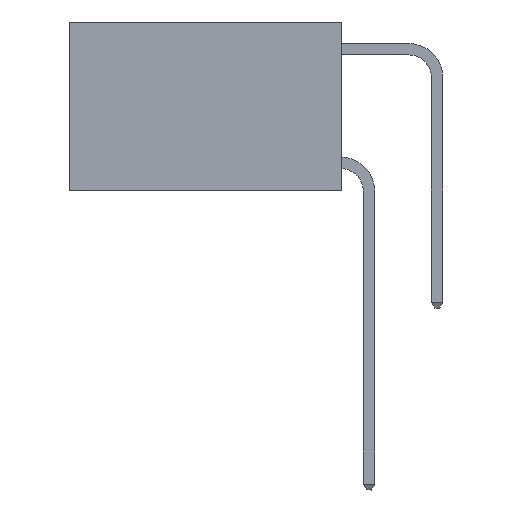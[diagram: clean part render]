
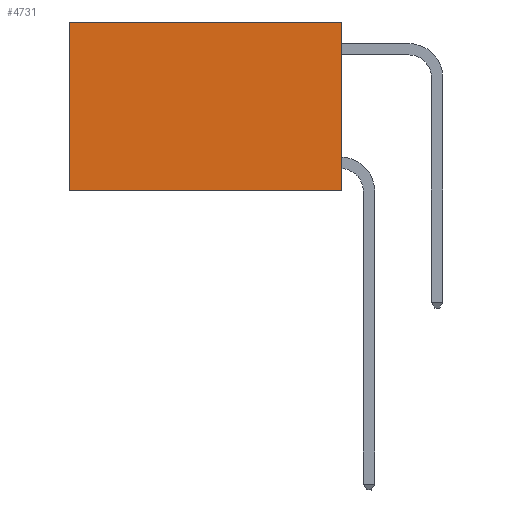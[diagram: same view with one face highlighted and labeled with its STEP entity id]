
A CAD part, left-side view. The second image highlights one B-rep face of the part: STEP entity #4731.
In plain terms, the highlighted planar face has unit normal (-1, 0, 0).
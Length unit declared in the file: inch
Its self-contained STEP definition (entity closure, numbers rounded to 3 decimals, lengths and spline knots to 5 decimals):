
#250 = VECTOR ( 'NONE', #14579, 39.37008 ) ;
#752 = CARTESIAN_POINT ( 'NONE',  ( 0.2625, 0., 0. ) ) ;
#1429 = CARTESIAN_POINT ( 'NONE',  ( 0.2625, 0.6, 0. ) ) ;
#2298 = EDGE_CURVE ( 'NONE', #16656, #6721, #19613, .T. ) ;
#3816 = CARTESIAN_POINT ( 'NONE',  ( 0.2625, 0., 0. ) ) ;
#4024 = VERTEX_POINT ( 'NONE', #13666 ) ;
#4731 = ADVANCED_FACE ( 'NONE', ( #18735 ), #27846, .F. ) ;
#6328 = CARTESIAN_POINT ( 'NONE',  ( 0.2625, 0., -0.37 ) ) ;
#6510 = AXIS2_PLACEMENT_3D ( 'NONE', #752, #19000, #16621 ) ;
#6721 = VERTEX_POINT ( 'NONE', #23463 ) ;
#8429 = DIRECTION ( 'NONE',  ( 0., 1., 0. ) ) ;
#9135 = EDGE_CURVE ( 'NONE', #6721, #4024, #15319, .T. ) ;
#9207 = EDGE_CURVE ( 'NONE', #16656, #15273, #22321, .T. ) ;
#9357 = VECTOR ( 'NONE', #17318, 39.37008 ) ;
#9696 = EDGE_LOOP ( 'NONE', ( #26089, #19393, #28889, #17922 ) ) ;
#10549 = CARTESIAN_POINT ( 'NONE',  ( 0.2625, 0., -0.37 ) ) ;
#12147 = LINE ( 'NONE', #10549, #13561 ) ;
#12795 = CARTESIAN_POINT ( 'NONE',  ( 0.2625, 0., 0. ) ) ;
#13561 = VECTOR ( 'NONE', #17631, 39.37008 ) ;
#13666 = CARTESIAN_POINT ( 'NONE',  ( 0.2625, 0.6, -0.37 ) ) ;
#14579 = DIRECTION ( 'NONE',  ( 0., 0., -1. ) ) ;
#15273 = VERTEX_POINT ( 'NONE', #6328 ) ;
#15319 = LINE ( 'NONE', #1429, #250 ) ;
#16621 = DIRECTION ( 'NONE',  ( 0., 0., -1. ) ) ;
#16656 = VERTEX_POINT ( 'NONE', #3816 ) ;
#17318 = DIRECTION ( 'NONE',  ( 0., 0., -1. ) ) ;
#17631 = DIRECTION ( 'NONE',  ( 0., 1., 0. ) ) ;
#17922 = ORIENTED_EDGE ( 'NONE', *, *, #2298, .T. ) ;
#18735 = FACE_OUTER_BOUND ( 'NONE', #9696, .T. ) ;
#18859 = EDGE_CURVE ( 'NONE', #15273, #4024, #12147, .T. ) ;
#19000 = DIRECTION ( 'NONE',  ( 1., 0., 0. ) ) ;
#19393 = ORIENTED_EDGE ( 'NONE', *, *, #18859, .F. ) ;
#19427 = CARTESIAN_POINT ( 'NONE',  ( 0.2625, 0., 0. ) ) ;
#19613 = LINE ( 'NONE', #19427, #25185 ) ;
#22321 = LINE ( 'NONE', #12795, #9357 ) ;
#23463 = CARTESIAN_POINT ( 'NONE',  ( 0.2625, 0.6, 0. ) ) ;
#25185 = VECTOR ( 'NONE', #8429, 39.37008 ) ;
#26089 = ORIENTED_EDGE ( 'NONE', *, *, #9135, .T. ) ;
#27846 = PLANE ( 'NONE',  #6510 ) ;
#28889 = ORIENTED_EDGE ( 'NONE', *, *, #9207, .F. ) ;
